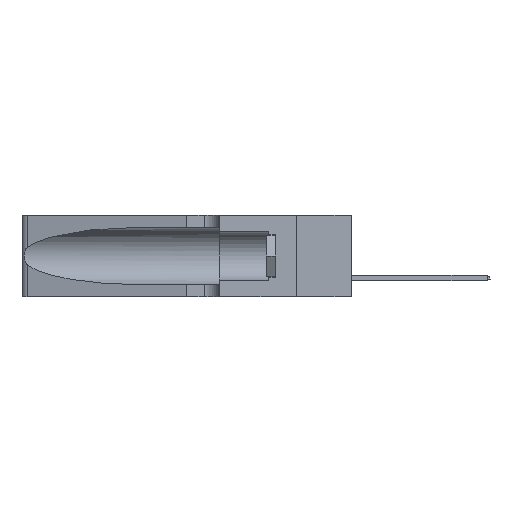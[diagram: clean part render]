
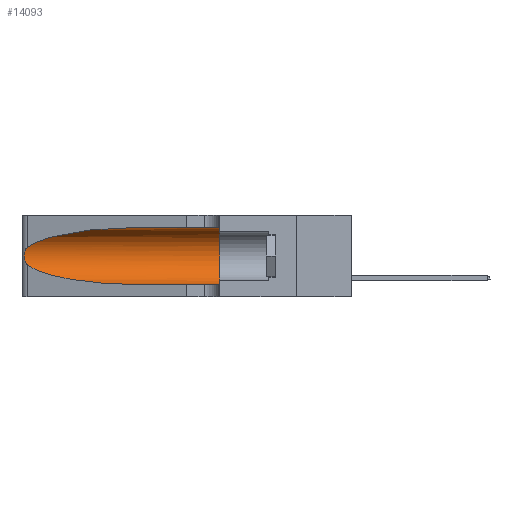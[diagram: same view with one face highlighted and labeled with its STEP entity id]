
A CAD part, left-side view. The second image highlights one B-rep face of the part: STEP entity #14093.
In plain terms, the highlighted cylindrical face has radius 3.308 mm (diameter 6.617 mm), a partial arc.
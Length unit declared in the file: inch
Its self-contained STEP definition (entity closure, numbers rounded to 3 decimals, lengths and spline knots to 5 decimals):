
#148 = EDGE_CURVE ( 'NONE', #3502, #4421, #24434, .T. ) ;
#268 = ORIENTED_EDGE ( 'NONE', *, *, #1760, .T. ) ;
#975 =( BOUNDED_CURVE ( )  B_SPLINE_CURVE ( 3, ( #9230, #24679, #14372, #27838 ),
 .UNSPECIFIED., .F., .T. ) 
 B_SPLINE_CURVE_WITH_KNOTS ( ( 4, 4 ),
 ( 1.5708, 2.84003 ),
 .UNSPECIFIED. ) 
 CURVE ( )  GEOMETRIC_REPRESENTATION_ITEM ( )  RATIONAL_B_SPLINE_CURVE ( ( 1., 0.87, 0.87, 1. ) ) 
 REPRESENTATION_ITEM ( '' )  );
#1691 = LINE ( 'NONE', #25847, #17093 ) ;
#1760 = EDGE_CURVE ( 'NONE', #26975, #5460, #975, .T. ) ;
#2378 = LINE ( 'NONE', #10156, #9411 ) ;
#3245 = DIRECTION ( 'NONE',  ( 0., -1., 0. ) ) ;
#3366 = DIRECTION ( 'NONE',  ( 0., 0., 1. ) ) ;
#3502 = VERTEX_POINT ( 'NONE', #24452 ) ;
#4335 = CARTESIAN_POINT ( 'NONE',  ( 0.2373, 1.15595, 0.08982 ) ) ;
#4421 = VERTEX_POINT ( 'NONE', #4755 ) ;
#4755 = CARTESIAN_POINT ( 'NONE',  ( 0.1305, 0.35, 0.05475 ) ) ;
#5460 = VERTEX_POINT ( 'NONE', #31848 ) ;
#6796 = AXIS2_PLACEMENT_3D ( 'NONE', #18349, #31702, #30792 ) ;
#8716 = CARTESIAN_POINT ( 'NONE',  ( 0.25787, 1.23484, 0.2124 ) ) ;
#8943 = CARTESIAN_POINT ( 'NONE',  ( 0.25487, 1.22718, 0.14631 ) ) ;
#9158 = EDGE_CURVE ( 'NONE', #26975, #3502, #2378, .T. ) ;
#9230 = CARTESIAN_POINT ( 'NONE',  ( 0.1305, 0.72297, 0.31525 ) ) ;
#9411 = VECTOR ( 'NONE', #18373, 39.37008 ) ;
#10005 = CARTESIAN_POINT ( 'NONE',  ( 0.1305, 0.72297, 0.31525 ) ) ;
#10156 = CARTESIAN_POINT ( 'NONE',  ( 0.1305, 1.61858, 0.31525 ) ) ;
#10841 = CARTESIAN_POINT ( 'NONE',  ( 0.25487, 1.22718, 0.22369 ) ) ;
#11413 = CARTESIAN_POINT ( 'NONE',  ( 0.26075, 1.23896, 0.19203 ) ) ;
#11568 = ORIENTED_EDGE ( 'NONE', *, *, #15298, .T. ) ;
#11644 = CARTESIAN_POINT ( 'NONE',  ( 0.25639, 1.23184, 0.21858 ) ) ;
#11900 = CARTESIAN_POINT ( 'NONE',  ( 0.1305, 0.72297, 0.05475 ) ) ;
#13389 = CARTESIAN_POINT ( 'NONE',  ( 0.25487, 1.22718, 0.14631 ) ) ;
#13511 = CARTESIAN_POINT ( 'NONE',  ( 0.25854, 1.2359, 0.20912 ) ) ;
#14093 = ADVANCED_FACE ( 'NONE', ( #25527 ), #27583, .F. ) ;
#14372 = CARTESIAN_POINT ( 'NONE',  ( 0.2373, 1.15595, 0.28018 ) ) ;
#15298 = EDGE_CURVE ( 'NONE', #31773, #4421, #1691, .T. ) ;
#16066 = CARTESIAN_POINT ( 'NONE',  ( 0.25555, 1.22993, 0.14849 ) ) ;
#16684 = EDGE_CURVE ( 'NONE', #28806, #31773, #29347, .T. ) ;
#16865 = CARTESIAN_POINT ( 'NONE',  ( 0.25856, 1.23593, 0.16098 ) ) ;
#17093 = VECTOR ( 'NONE', #3245, 39.37008 ) ;
#18349 = CARTESIAN_POINT ( 'NONE',  ( 0.1305, 1.61858, 0.185 ) ) ;
#18373 = DIRECTION ( 'NONE',  ( 0., -1., 0. ) ) ;
#19036 = ORIENTED_EDGE ( 'NONE', *, *, #32748, .T. ) ;
#19641 = CARTESIAN_POINT ( 'NONE',  ( 0.1305, 0.35, 0.185 ) ) ;
#20003 = CARTESIAN_POINT ( 'NONE',  ( 0.25487, 1.22718, 0.14631 ) ) ;
#20301 = ORIENTED_EDGE ( 'NONE', *, *, #148, .F. ) ;
#21057 = ORIENTED_EDGE ( 'NONE', *, *, #9158, .F. ) ;
#21292 = B_SPLINE_CURVE_WITH_KNOTS ( 'NONE', 3,
 ( #10841, #29407, #11644, #8716, #13511, #22190, #11413, #27432, #32756, #16865, #22310, #30215, #16066, #8943 ),
 .UNSPECIFIED., .F., .F.,
 ( 4, 2, 2, 2, 2, 2, 4 ),
 ( 0., 0.00027, 0.00053, 0.00107, 0.0016, 0.00187, 0.00214 ),
 .UNSPECIFIED. ) ;
#22190 = CARTESIAN_POINT ( 'NONE',  ( 0.26018, 1.23835, 0.19895 ) ) ;
#22310 = CARTESIAN_POINT ( 'NONE',  ( 0.25789, 1.23486, 0.15765 ) ) ;
#22919 = CARTESIAN_POINT ( 'NONE',  ( 0.18966, 0.96281, 0.05475 ) ) ;
#24398 = ORIENTED_EDGE ( 'NONE', *, *, #16684, .T. ) ;
#24434 = CIRCLE ( 'NONE', #29584, 0.13025 ) ;
#24452 = CARTESIAN_POINT ( 'NONE',  ( 0.1305, 0.35, 0.31525 ) ) ;
#24679 = CARTESIAN_POINT ( 'NONE',  ( 0.18966, 0.96281, 0.31525 ) ) ;
#24683 = EDGE_LOOP ( 'NONE', ( #268, #19036, #24398, #11568, #20301, #21057 ) ) ;
#25527 = FACE_OUTER_BOUND ( 'NONE', #24683, .T. ) ;
#25645 = CARTESIAN_POINT ( 'NONE',  ( 0.1305, 0.72297, 0.05475 ) ) ;
#25847 = CARTESIAN_POINT ( 'NONE',  ( 0.1305, 1.61858, 0.05475 ) ) ;
#26975 = VERTEX_POINT ( 'NONE', #10005 ) ;
#27432 = CARTESIAN_POINT ( 'NONE',  ( 0.26075, 1.23896, 0.178 ) ) ;
#27583 = CYLINDRICAL_SURFACE ( 'NONE', #6796, 0.13025 ) ;
#27838 = CARTESIAN_POINT ( 'NONE',  ( 0.25487, 1.22718, 0.22369 ) ) ;
#28806 = VERTEX_POINT ( 'NONE', #13389 ) ;
#29347 =( BOUNDED_CURVE ( )  B_SPLINE_CURVE ( 3, ( #20003, #4335, #22919, #11900 ),
 .UNSPECIFIED., .F., .F. ) 
 B_SPLINE_CURVE_WITH_KNOTS ( ( 4, 4 ),
 ( 3.44316, 4.71239 ),
 .UNSPECIFIED. ) 
 CURVE ( )  GEOMETRIC_REPRESENTATION_ITEM ( )  RATIONAL_B_SPLINE_CURVE ( ( 1., 0.87, 0.87, 1. ) ) 
 REPRESENTATION_ITEM ( '' )  );
#29407 = CARTESIAN_POINT ( 'NONE',  ( 0.25555, 1.22994, 0.2215 ) ) ;
#29584 = AXIS2_PLACEMENT_3D ( 'NONE', #19641, #32532, #3366 ) ;
#30215 = CARTESIAN_POINT ( 'NONE',  ( 0.25639, 1.23186, 0.15144 ) ) ;
#30792 = DIRECTION ( 'NONE',  ( 0., 0., -1. ) ) ;
#31702 = DIRECTION ( 'NONE',  ( 0., -1., 0. ) ) ;
#31773 = VERTEX_POINT ( 'NONE', #25645 ) ;
#31848 = CARTESIAN_POINT ( 'NONE',  ( 0.25487, 1.22718, 0.22369 ) ) ;
#32532 = DIRECTION ( 'NONE',  ( 0., 1., 0. ) ) ;
#32748 = EDGE_CURVE ( 'NONE', #5460, #28806, #21292, .T. ) ;
#32756 = CARTESIAN_POINT ( 'NONE',  ( 0.26017, 1.23833, 0.17102 ) ) ;
